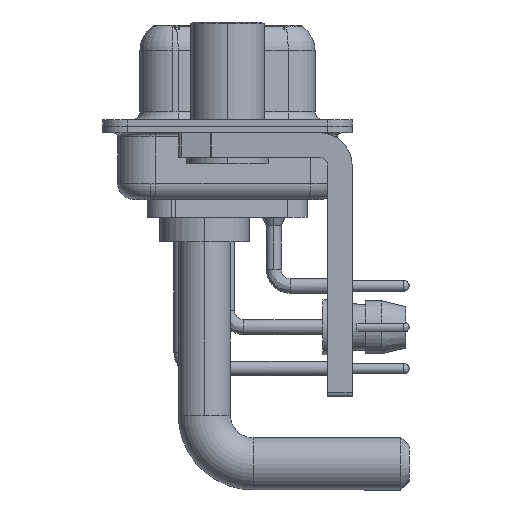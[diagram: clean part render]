
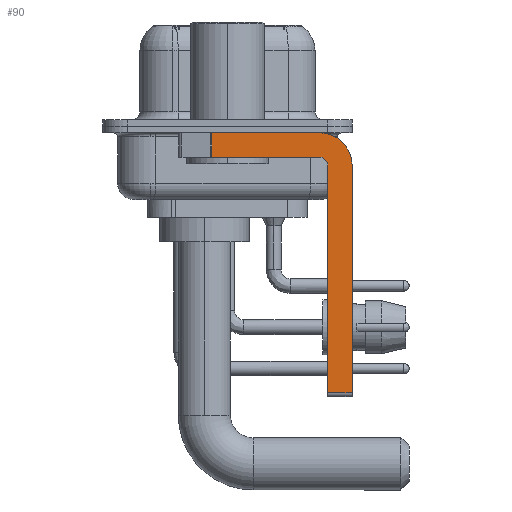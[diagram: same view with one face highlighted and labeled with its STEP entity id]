
A CAD part, left-side view. The second image highlights one B-rep face of the part: STEP entity #90.
In plain terms, the highlighted planar face has unit normal (-1, 0, 0).
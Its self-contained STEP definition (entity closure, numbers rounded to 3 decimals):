
#90 = ADVANCED_FACE ( 'NONE', ( #32572 ), #26920, .F. ) ;
#361 = DIRECTION ( 'NONE',  ( 0., 0., 1. ) ) ;
#530 = ORIENTED_EDGE ( 'NONE', *, *, #26249, .F. ) ;
#1391 = CARTESIAN_POINT ( 'NONE',  ( -2.9, -5.65, -16.35 ) ) ;
#1600 = CARTESIAN_POINT ( 'NONE',  ( -2.9, 0.978, -1.9 ) ) ;
#1771 = EDGE_CURVE ( 'NONE', #7692, #26043, #27949, .T. ) ;
#1910 = AXIS2_PLACEMENT_3D ( 'NONE', #11998, #16998, #361 ) ;
#1937 = DIRECTION ( 'NONE',  ( 0., 0., -1. ) ) ;
#4144 = CARTESIAN_POINT ( 'NONE',  ( -2.9, -5.65, -2.4 ) ) ;
#4358 = VECTOR ( 'NONE', #14503, 1000. ) ;
#4455 = AXIS2_PLACEMENT_3D ( 'NONE', #4144, #14284, #10627 ) ;
#4616 = AXIS2_PLACEMENT_3D ( 'NONE', #22549, #27057, #1937 ) ;
#4618 = CARTESIAN_POINT ( 'NONE',  ( -2.9, 0.978, -1.9 ) ) ;
#4810 = VECTOR ( 'NONE', #10231, 1000. ) ;
#5113 = ORIENTED_EDGE ( 'NONE', *, *, #21728, .F. ) ;
#5479 = CARTESIAN_POINT ( 'NONE',  ( -2.9, -6.15, -16.35 ) ) ;
#5785 = CARTESIAN_POINT ( 'NONE',  ( -2.9, -5.65, -1.9 ) ) ;
#7239 = LINE ( 'NONE', #23014, #4810 ) ;
#7465 = VECTOR ( 'NONE', #18394, 1000. ) ;
#7692 = VERTEX_POINT ( 'NONE', #11371 ) ;
#8263 = CARTESIAN_POINT ( 'NONE',  ( -2.9, -5.65, -1.9 ) ) ;
#9923 = ORIENTED_EDGE ( 'NONE', *, *, #24597, .T. ) ;
#10231 = DIRECTION ( 'NONE',  ( 0., -1., 0. ) ) ;
#10627 = DIRECTION ( 'NONE',  ( 0., 0., -1. ) ) ;
#11238 = ORIENTED_EDGE ( 'NONE', *, *, #30444, .F. ) ;
#11348 = VERTEX_POINT ( 'NONE', #30677 ) ;
#11371 = CARTESIAN_POINT ( 'NONE',  ( -2.9, -5.65, -0.4 ) ) ;
#11507 = CARTESIAN_POINT ( 'NONE',  ( -2.9, 0.978, -0.4 ) ) ;
#11998 = CARTESIAN_POINT ( 'NONE',  ( -2.9, -5.65, -2.4 ) ) ;
#12467 = VECTOR ( 'NONE', #15932, 1000. ) ;
#13181 = CARTESIAN_POINT ( 'NONE',  ( -2.9, -6.15, -16.6 ) ) ;
#14284 = DIRECTION ( 'NONE',  ( 1., 0., 0. ) ) ;
#14503 = DIRECTION ( 'NONE',  ( 0., -1., 0. ) ) ;
#14717 = LINE ( 'NONE', #1600, #27682 ) ;
#14952 = ORIENTED_EDGE ( 'NONE', *, *, #23512, .T. ) ;
#15932 = DIRECTION ( 'NONE',  ( 0., 0., -1. ) ) ;
#16776 = VERTEX_POINT ( 'NONE', #31794 ) ;
#16998 = DIRECTION ( 'NONE',  ( -1., 0., 0. ) ) ;
#17964 = EDGE_LOOP ( 'NONE', ( #28797, #9923, #5113, #11238, #530, #14952, #23909, #24483 ) ) ;
#18142 = VERTEX_POINT ( 'NONE', #11507 ) ;
#18394 = DIRECTION ( 'NONE',  ( 0., 1., 0. ) ) ;
#19817 = VECTOR ( 'NONE', #23642, 1000. ) ;
#20599 = VERTEX_POINT ( 'NONE', #4618 ) ;
#20882 = LINE ( 'NONE', #8263, #7465 ) ;
#21728 = EDGE_CURVE ( 'NONE', #22876, #20599, #20882, .T. ) ;
#21880 = EDGE_CURVE ( 'NONE', #18142, #7692, #7239, .T. ) ;
#22549 = CARTESIAN_POINT ( 'NONE',  ( -2.9, -5.65, -2.4 ) ) ;
#22876 = VERTEX_POINT ( 'NONE', #5785 ) ;
#23014 = CARTESIAN_POINT ( 'NONE',  ( -2.9, 3., -0.4 ) ) ;
#23311 = LINE ( 'NONE', #13181, #19817 ) ;
#23512 = EDGE_CURVE ( 'NONE', #29994, #11348, #23838, .T. ) ;
#23642 = DIRECTION ( 'NONE',  ( 0., 0., 1. ) ) ;
#23838 = LINE ( 'NONE', #1391, #4358 ) ;
#23909 = ORIENTED_EDGE ( 'NONE', *, *, #29890, .F. ) ;
#24483 = ORIENTED_EDGE ( 'NONE', *, *, #1771, .F. ) ;
#24597 = EDGE_CURVE ( 'NONE', #18142, #20599, #14717, .T. ) ;
#26043 = VERTEX_POINT ( 'NONE', #29160 ) ;
#26249 = EDGE_CURVE ( 'NONE', #29994, #16776, #23311, .T. ) ;
#26920 = PLANE ( 'NONE',  #4455 ) ;
#27057 = DIRECTION ( 'NONE',  ( 1., 0., 0. ) ) ;
#27682 = VECTOR ( 'NONE', #29682, 1000. ) ;
#27922 = CIRCLE ( 'NONE', #1910, 0.5 ) ;
#27949 = CIRCLE ( 'NONE', #4616, 2. ) ;
#28797 = ORIENTED_EDGE ( 'NONE', *, *, #21880, .F. ) ;
#28886 = LINE ( 'NONE', #31062, #12467 ) ;
#29160 = CARTESIAN_POINT ( 'NONE',  ( -2.9, -7.65, -2.4 ) ) ;
#29682 = DIRECTION ( 'NONE',  ( 0., 0., -1. ) ) ;
#29890 = EDGE_CURVE ( 'NONE', #26043, #11348, #28886, .T. ) ;
#29994 = VERTEX_POINT ( 'NONE', #5479 ) ;
#30444 = EDGE_CURVE ( 'NONE', #16776, #22876, #27922, .T. ) ;
#30677 = CARTESIAN_POINT ( 'NONE',  ( -2.9, -7.65, -16.35 ) ) ;
#31062 = CARTESIAN_POINT ( 'NONE',  ( -2.9, -7.65, -2.4 ) ) ;
#31794 = CARTESIAN_POINT ( 'NONE',  ( -2.9, -6.15, -2.4 ) ) ;
#32572 = FACE_OUTER_BOUND ( 'NONE', #17964, .T. ) ;
